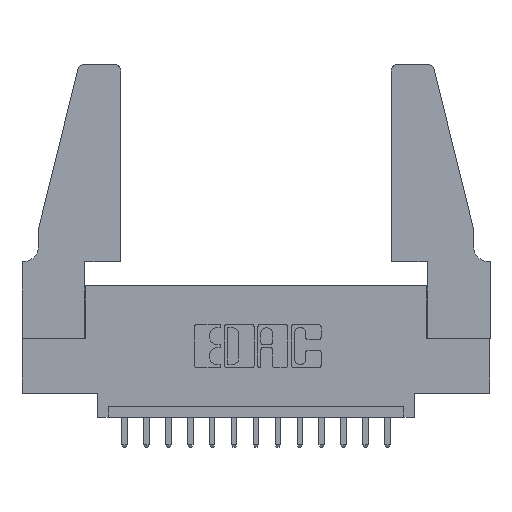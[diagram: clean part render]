
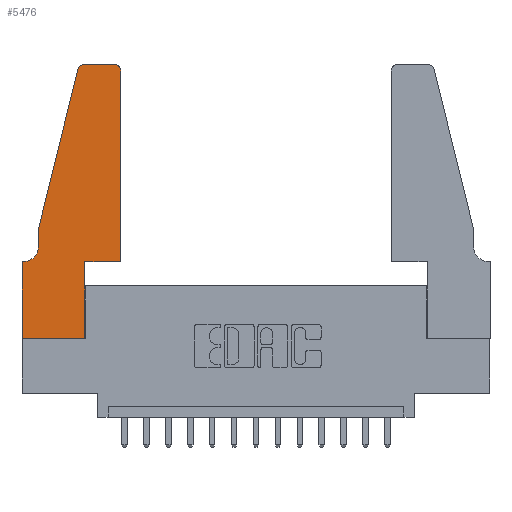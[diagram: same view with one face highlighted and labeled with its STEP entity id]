
A CAD part, top view. The second image highlights one B-rep face of the part: STEP entity #5476.
In plain terms, the highlighted planar face has unit normal (0, 0, 1).
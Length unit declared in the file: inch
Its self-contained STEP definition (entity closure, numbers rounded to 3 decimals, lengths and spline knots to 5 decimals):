
#24 = ORIENTED_EDGE ( 'NONE', *, *, #1209, .T. ) ;
#149 = LINE ( 'NONE', #10442, #9055 ) ;
#487 = VECTOR ( 'NONE', #14624, 39.37008 ) ;
#748 = CIRCLE ( 'NONE', #8271, 0.07 ) ;
#950 = CARTESIAN_POINT ( 'NONE',  ( 0.0755, 0.5, 0.37 ) ) ;
#1113 = AXIS2_PLACEMENT_3D ( 'NONE', #10200, #1592, #12483 ) ;
#1209 = EDGE_CURVE ( 'NONE', #3985, #6070, #14099, .T. ) ;
#1315 = AXIS2_PLACEMENT_3D ( 'NONE', #2868, #7633, #6587 ) ;
#1592 = DIRECTION ( 'NONE',  ( 0., 0., 1. ) ) ;
#1655 = LINE ( 'NONE', #5913, #487 ) ;
#2093 = VERTEX_POINT ( 'NONE', #15030 ) ;
#2136 = CARTESIAN_POINT ( 'NONE',  ( 0.2605, 1.25, 0.37 ) ) ;
#2194 = ORIENTED_EDGE ( 'NONE', *, *, #2685, .T. ) ;
#2488 = VECTOR ( 'NONE', #5245, 39.37008 ) ;
#2595 = CARTESIAN_POINT ( 'NONE',  ( 0.0755, 0.5, 0.37 ) ) ;
#2663 = CARTESIAN_POINT ( 'NONE',  ( 0., 0.35, 0.37 ) ) ;
#2685 = EDGE_CURVE ( 'NONE', #9683, #7869, #149, .T. ) ;
#2705 = VECTOR ( 'NONE', #15924, 39.37008 ) ;
#2868 = CARTESIAN_POINT ( 'NONE',  ( 0.4205, 1.22, 0.37 ) ) ;
#3215 = VERTEX_POINT ( 'NONE', #6455 ) ;
#3342 = CARTESIAN_POINT ( 'NONE',  ( 0.0755, 0.35, 0.37 ) ) ;
#3384 = VERTEX_POINT ( 'NONE', #14944 ) ;
#3648 = ORIENTED_EDGE ( 'NONE', *, *, #8647, .T. ) ;
#3743 = PLANE ( 'NONE',  #7424 ) ;
#3985 = VERTEX_POINT ( 'NONE', #13496 ) ;
#4382 = ORIENTED_EDGE ( 'NONE', *, *, #14279, .T. ) ;
#4542 = CIRCLE ( 'NONE', #1113, 0.03 ) ;
#4586 = LINE ( 'NONE', #8849, #2488 ) ;
#4899 = DIRECTION ( 'NONE',  ( 1., 0., 0. ) ) ;
#4943 = LINE ( 'NONE', #8513, #13869 ) ;
#5056 = DIRECTION ( 'NONE',  ( 1., 0., 0. ) ) ;
#5081 = ORIENTED_EDGE ( 'NONE', *, *, #12079, .T. ) ;
#5144 = CARTESIAN_POINT ( 'NONE',  ( 0.0755, 0.42, 0.37 ) ) ;
#5245 = DIRECTION ( 'NONE',  ( 0., 1., 0. ) ) ;
#5476 = ADVANCED_FACE ( 'NONE', ( #9707 ), #3743, .T. ) ;
#5725 = EDGE_CURVE ( 'NONE', #9932, #3384, #748, .T. ) ;
#5913 = CARTESIAN_POINT ( 'NONE',  ( 0.4505, 0.35, 0.37 ) ) ;
#5988 = ORIENTED_EDGE ( 'NONE', *, *, #11470, .T. ) ;
#6070 = VERTEX_POINT ( 'NONE', #8428 ) ;
#6274 = EDGE_CURVE ( 'NONE', #12992, #9683, #4586, .T. ) ;
#6455 = CARTESIAN_POINT ( 'NONE',  ( 0.284, 1.25, 0.37 ) ) ;
#6587 = DIRECTION ( 'NONE',  ( 1., 0., 0. ) ) ;
#6588 = ORIENTED_EDGE ( 'NONE', *, *, #15635, .T. ) ;
#6678 = EDGE_CURVE ( 'NONE', #13351, #14877, #4943, .T. ) ;
#6955 = LINE ( 'NONE', #950, #2705 ) ;
#7424 = AXIS2_PLACEMENT_3D ( 'NONE', #2663, #8838, #5056 ) ;
#7633 = DIRECTION ( 'NONE',  ( 0., 0., 1. ) ) ;
#7680 = VERTEX_POINT ( 'NONE', #11835 ) ;
#7743 = VECTOR ( 'NONE', #15733, 39.37008 ) ;
#7869 = VERTEX_POINT ( 'NONE', #9889 ) ;
#8164 = DIRECTION ( 'NONE',  ( 1., 0., 0. ) ) ;
#8262 = ORIENTED_EDGE ( 'NONE', *, *, #14725, .T. ) ;
#8271 = AXIS2_PLACEMENT_3D ( 'NONE', #11580, #14263, #12959 ) ;
#8428 = CARTESIAN_POINT ( 'NONE',  ( 0.0755, 0.5, 0.37 ) ) ;
#8513 = CARTESIAN_POINT ( 'NONE',  ( 0., 0., 0.37 ) ) ;
#8647 = EDGE_CURVE ( 'NONE', #3384, #13351, #11314, .T. ) ;
#8768 = CARTESIAN_POINT ( 'NONE',  ( 0.2865, 0., 0.37 ) ) ;
#8838 = DIRECTION ( 'NONE',  ( 0., 0., 1. ) ) ;
#8849 = CARTESIAN_POINT ( 'NONE',  ( 0.2865, 0.35, 0.37 ) ) ;
#8897 = LINE ( 'NONE', #2136, #7743 ) ;
#9055 = VECTOR ( 'NONE', #8164, 39.37008 ) ;
#9550 = DIRECTION ( 'NONE',  ( 0., -1., 0. ) ) ;
#9683 = VERTEX_POINT ( 'NONE', #15988 ) ;
#9707 = FACE_OUTER_BOUND ( 'NONE', #10591, .T. ) ;
#9889 = CARTESIAN_POINT ( 'NONE',  ( 0.4505, 0.35, 0.37 ) ) ;
#9932 = VERTEX_POINT ( 'NONE', #5144 ) ;
#10106 = VECTOR ( 'NONE', #4899, 39.37008 ) ;
#10200 = CARTESIAN_POINT ( 'NONE',  ( 0.284, 1.22, 0.37 ) ) ;
#10442 = CARTESIAN_POINT ( 'NONE',  ( 0.4505, 0.35, 0.37 ) ) ;
#10545 = VECTOR ( 'NONE', #11919, 39.37008 ) ;
#10591 = EDGE_LOOP ( 'NONE', ( #15435, #4382, #24, #5081, #10906, #3648, #14926, #5988, #12369, #2194, #8262, #6588 ) ) ;
#10834 = VECTOR ( 'NONE', #12361, 39.37008 ) ;
#10906 = ORIENTED_EDGE ( 'NONE', *, *, #5725, .T. ) ;
#11314 = LINE ( 'NONE', #3342, #10545 ) ;
#11470 = EDGE_CURVE ( 'NONE', #14877, #12992, #13362, .T. ) ;
#11580 = CARTESIAN_POINT ( 'NONE',  ( 0.0055, 0.42, 0.37 ) ) ;
#11835 = CARTESIAN_POINT ( 'NONE',  ( 0.4505, 1.22, 0.37 ) ) ;
#11919 = DIRECTION ( 'NONE',  ( -1., 0., 0. ) ) ;
#12079 = EDGE_CURVE ( 'NONE', #6070, #9932, #6955, .T. ) ;
#12166 = CARTESIAN_POINT ( 'NONE',  ( 0., 0., 0.37 ) ) ;
#12361 = DIRECTION ( 'NONE',  ( -0.239, -0.971, 0. ) ) ;
#12369 = ORIENTED_EDGE ( 'NONE', *, *, #6274, .T. ) ;
#12397 = EDGE_CURVE ( 'NONE', #2093, #3215, #8897, .T. ) ;
#12483 = DIRECTION ( 'NONE',  ( 1., 0., 0. ) ) ;
#12726 = CIRCLE ( 'NONE', #1315, 0.03 ) ;
#12959 = DIRECTION ( 'NONE',  ( -1., 0., 0. ) ) ;
#12992 = VERTEX_POINT ( 'NONE', #8768 ) ;
#13351 = VERTEX_POINT ( 'NONE', #14532 ) ;
#13362 = LINE ( 'NONE', #14438, #10106 ) ;
#13496 = CARTESIAN_POINT ( 'NONE',  ( 0.25487, 1.22718, 0.37 ) ) ;
#13869 = VECTOR ( 'NONE', #9550, 39.37008 ) ;
#14099 = LINE ( 'NONE', #2595, #10834 ) ;
#14263 = DIRECTION ( 'NONE',  ( 0., 0., -1. ) ) ;
#14279 = EDGE_CURVE ( 'NONE', #3215, #3985, #4542, .T. ) ;
#14438 = CARTESIAN_POINT ( 'NONE',  ( 0., 0., 0.37 ) ) ;
#14532 = CARTESIAN_POINT ( 'NONE',  ( 0., 0.35, 0.37 ) ) ;
#14624 = DIRECTION ( 'NONE',  ( 0., 1., 0. ) ) ;
#14725 = EDGE_CURVE ( 'NONE', #7869, #7680, #1655, .T. ) ;
#14877 = VERTEX_POINT ( 'NONE', #12166 ) ;
#14926 = ORIENTED_EDGE ( 'NONE', *, *, #6678, .T. ) ;
#14944 = CARTESIAN_POINT ( 'NONE',  ( 0.0055, 0.35, 0.37 ) ) ;
#15030 = CARTESIAN_POINT ( 'NONE',  ( 0.4205, 1.25, 0.37 ) ) ;
#15435 = ORIENTED_EDGE ( 'NONE', *, *, #12397, .T. ) ;
#15635 = EDGE_CURVE ( 'NONE', #7680, #2093, #12726, .T. ) ;
#15733 = DIRECTION ( 'NONE',  ( -1., 0., 0. ) ) ;
#15924 = DIRECTION ( 'NONE',  ( 0., -1., 0. ) ) ;
#15988 = CARTESIAN_POINT ( 'NONE',  ( 0.2865, 0.35, 0.37 ) ) ;
